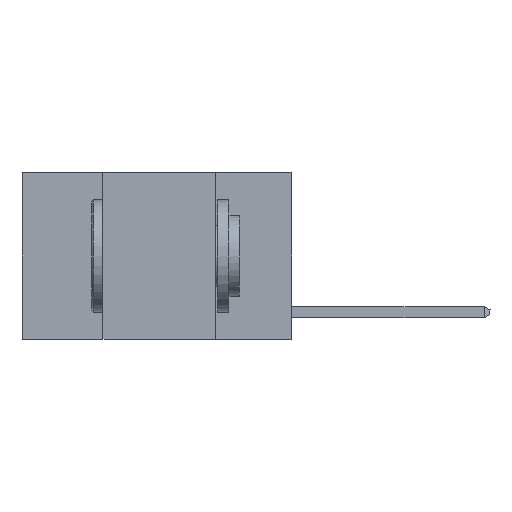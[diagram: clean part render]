
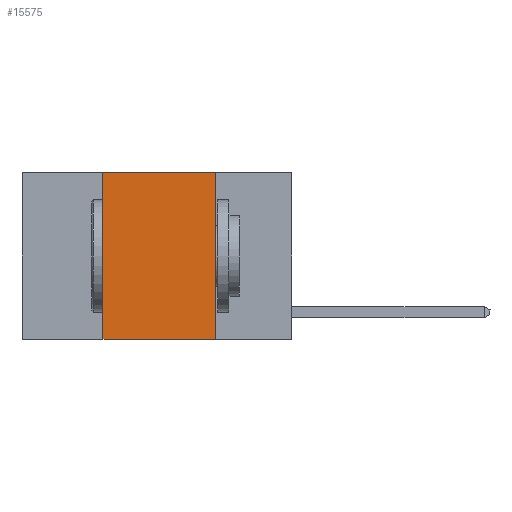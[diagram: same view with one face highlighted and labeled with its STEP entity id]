
A CAD part, left-side view. The second image highlights one B-rep face of the part: STEP entity #15575.
In plain terms, the highlighted planar face has unit normal (-1, 0, 0).
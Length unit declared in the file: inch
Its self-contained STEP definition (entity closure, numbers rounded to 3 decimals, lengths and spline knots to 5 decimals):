
#661 = ORIENTED_EDGE ( 'NONE', *, *, #11239, .T. ) ;
#985 = DIRECTION ( 'NONE',  ( 0., -1., 0. ) ) ;
#1275 = ORIENTED_EDGE ( 'NONE', *, *, #9776, .F. ) ;
#1668 = CARTESIAN_POINT ( 'NONE',  ( 0., 0.6, 0. ) ) ;
#3722 = PLANE ( 'NONE',  #22124 ) ;
#4983 = EDGE_CURVE ( 'NONE', #22413, #27261, #13600, .T. ) ;
#5859 = VECTOR ( 'NONE', #11531, 39.37008 ) ;
#7924 = DIRECTION ( 'NONE',  ( 0., 0., -1. ) ) ;
#7939 = EDGE_LOOP ( 'NONE', ( #1275, #13095, #16180, #661 ) ) ;
#9776 = EDGE_CURVE ( 'NONE', #27261, #24024, #13229, .T. ) ;
#11239 = EDGE_CURVE ( 'NONE', #28098, #24024, #21348, .T. ) ;
#11325 = CARTESIAN_POINT ( 'NONE',  ( 0., 0.17, 0. ) ) ;
#11531 = DIRECTION ( 'NONE',  ( 0., 0., 1. ) ) ;
#13095 = ORIENTED_EDGE ( 'NONE', *, *, #4983, .F. ) ;
#13229 = LINE ( 'NONE', #15723, #28242 ) ;
#13600 = LINE ( 'NONE', #1668, #22494 ) ;
#14117 = CARTESIAN_POINT ( 'NONE',  ( 0., 0.42, 0. ) ) ;
#14912 = VECTOR ( 'NONE', #985, 39.37008 ) ;
#15575 = ADVANCED_FACE ( 'NONE', ( #19708 ), #3722, .F. ) ;
#15723 = CARTESIAN_POINT ( 'NONE',  ( 0., 0.17, 0. ) ) ;
#16180 = ORIENTED_EDGE ( 'NONE', *, *, #17859, .F. ) ;
#17785 = CARTESIAN_POINT ( 'NONE',  ( 0., 0.42, -0.37 ) ) ;
#17859 = EDGE_CURVE ( 'NONE', #28098, #22413, #28017, .T. ) ;
#19708 = FACE_OUTER_BOUND ( 'NONE', #7939, .T. ) ;
#20341 = DIRECTION ( 'NONE',  ( 1., 0., 0. ) ) ;
#21033 = CARTESIAN_POINT ( 'NONE',  ( 0., 0.42, 0. ) ) ;
#21348 = LINE ( 'NONE', #28483, #14912 ) ;
#22124 = AXIS2_PLACEMENT_3D ( 'NONE', #29188, #20341, #7924 ) ;
#22413 = VERTEX_POINT ( 'NONE', #14117 ) ;
#22494 = VECTOR ( 'NONE', #25575, 39.37008 ) ;
#24024 = VERTEX_POINT ( 'NONE', #27321 ) ;
#25575 = DIRECTION ( 'NONE',  ( 0., -1., 0. ) ) ;
#27261 = VERTEX_POINT ( 'NONE', #11325 ) ;
#27321 = CARTESIAN_POINT ( 'NONE',  ( 0., 0.17, -0.37 ) ) ;
#27551 = DIRECTION ( 'NONE',  ( 0., 0., -1. ) ) ;
#28017 = LINE ( 'NONE', #21033, #5859 ) ;
#28098 = VERTEX_POINT ( 'NONE', #17785 ) ;
#28242 = VECTOR ( 'NONE', #27551, 39.37008 ) ;
#28483 = CARTESIAN_POINT ( 'NONE',  ( 0., 0.6, -0.37 ) ) ;
#29188 = CARTESIAN_POINT ( 'NONE',  ( 0., 0.6, 0. ) ) ;
